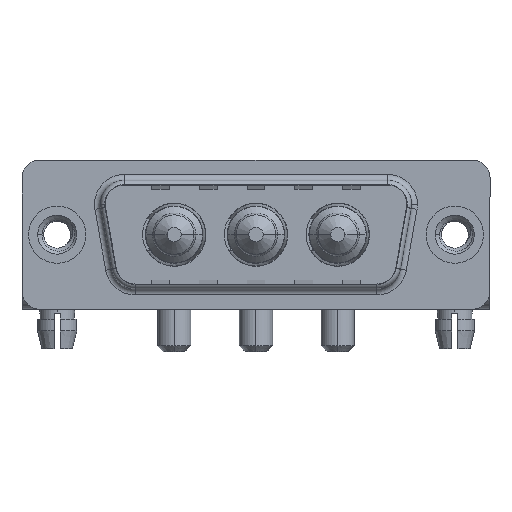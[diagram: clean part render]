
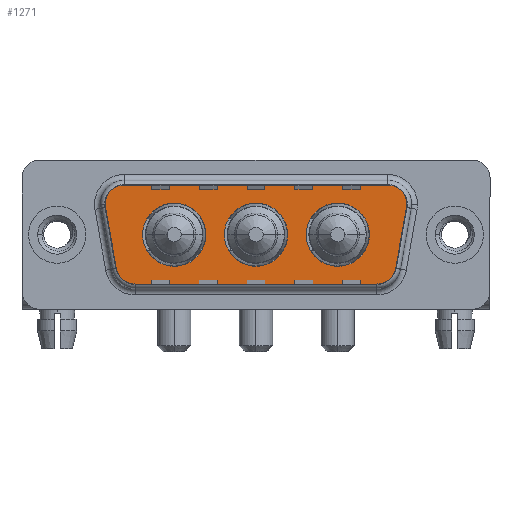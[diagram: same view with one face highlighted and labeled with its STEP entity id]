
A CAD part, top view. The second image highlights one B-rep face of the part: STEP entity #1271.
In plain terms, the highlighted planar face has unit normal (0, 0, 1).
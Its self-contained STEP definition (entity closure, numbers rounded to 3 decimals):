
#171 = VERTEX_POINT ( 'NONE', #11908 ) ;
#190 = CIRCLE ( 'NONE', #13988, 2.65 ) ;
#229 = DIRECTION ( 'NONE',  ( 0., 0., 1. ) ) ;
#417 = DIRECTION ( 'NONE',  ( 0.174, 0.985, 0. ) ) ;
#504 = CARTESIAN_POINT ( 'NONE',  ( 26.866, -2.9, 0. ) ) ;
#672 = CARTESIAN_POINT ( 'NONE',  ( 14., 0., 0. ) ) ;
#733 = CARTESIAN_POINT ( 'NONE',  ( 6.434, -4.9, 0. ) ) ;
#956 = ORIENTED_EDGE ( 'NONE', *, *, #7498, .F. ) ;
#975 = CARTESIAN_POINT ( 'NONE',  ( 5.411, 4.9, 0. ) ) ;
#1110 = EDGE_CURVE ( 'NONE', #8592, #13271, #4122, .T. ) ;
#1236 = LINE ( 'NONE', #11989, #11719 ) ;
#1271 = ADVANCED_FACE ( 'NONE', ( #8222, #8380, #13931, #12804 ), #3369, .T. ) ;
#1402 = VERTEX_POINT ( 'NONE', #4057 ) ;
#1997 = EDGE_LOOP ( 'NONE', ( #13132, #956 ) ) ;
#2053 = CIRCLE ( 'NONE', #6487, 2.65 ) ;
#2118 = VERTEX_POINT ( 'NONE', #13344 ) ;
#2180 = EDGE_CURVE ( 'NONE', #5391, #5598, #190, .T. ) ;
#2193 = ORIENTED_EDGE ( 'NONE', *, *, #7189, .F. ) ;
#2213 = DIRECTION ( 'NONE',  ( 1., 0., 0. ) ) ;
#2269 = CIRCLE ( 'NONE', #9163, 2. ) ;
#2426 = EDGE_CURVE ( 'NONE', #1402, #171, #12169, .T. ) ;
#2434 = CARTESIAN_POINT ( 'NONE',  ( 29.889, 2.9, 0. ) ) ;
#2473 = LINE ( 'NONE', #10884, #14920 ) ;
#2818 = AXIS2_PLACEMENT_3D ( 'NONE', #11722, #11875, #3447 ) ;
#2893 = ORIENTED_EDGE ( 'NONE', *, *, #14145, .T. ) ;
#3054 = CIRCLE ( 'NONE', #2818, 2.65 ) ;
#3228 = CARTESIAN_POINT ( 'NONE',  ( 20.85, 0., 0. ) ) ;
#3335 = DIRECTION ( 'NONE',  ( 0., 0., 1. ) ) ;
#3369 = PLANE ( 'NONE',  #13963 ) ;
#3447 = DIRECTION ( 'NONE',  ( 1., 0., 0. ) ) ;
#3895 = DIRECTION ( 'NONE',  ( 0., 0., 1. ) ) ;
#3896 = DIRECTION ( 'NONE',  ( 0., 0., 1. ) ) ;
#3942 = ORIENTED_EDGE ( 'NONE', *, *, #14695, .T. ) ;
#4038 = DIRECTION ( 'NONE',  ( 1., 0., 0. ) ) ;
#4057 = CARTESIAN_POINT ( 'NONE',  ( 28.836, -3.247, 0. ) ) ;
#4072 = DIRECTION ( 'NONE',  ( 0., 0., 1. ) ) ;
#4122 = CIRCLE ( 'NONE', #11779, 2. ) ;
#4148 = LINE ( 'NONE', #8859, #6401 ) ;
#4158 = VERTEX_POINT ( 'NONE', #733 ) ;
#4188 = EDGE_CURVE ( 'NONE', #4158, #2118, #4148, .T. ) ;
#4205 = CARTESIAN_POINT ( 'NONE',  ( 29.859, 2.553, 0. ) ) ;
#4219 = EDGE_CURVE ( 'NONE', #2118, #1402, #6156, .T. ) ;
#4650 = ORIENTED_EDGE ( 'NONE', *, *, #1110, .T. ) ;
#4975 = DIRECTION ( 'NONE',  ( 1., 0., 0. ) ) ;
#5220 = ORIENTED_EDGE ( 'NONE', *, *, #10240, .T. ) ;
#5391 = VERTEX_POINT ( 'NONE', #13229 ) ;
#5438 = VERTEX_POINT ( 'NONE', #10531 ) ;
#5490 = DIRECTION ( 'NONE',  ( 0., 0., 1. ) ) ;
#5598 = VERTEX_POINT ( 'NONE', #8586 ) ;
#5659 = DIRECTION ( 'NONE',  ( -1., 0., 0. ) ) ;
#5810 = DIRECTION ( 'NONE',  ( 1., 0., 0. ) ) ;
#5911 = VERTEX_POINT ( 'NONE', #7251 ) ;
#5928 = EDGE_LOOP ( 'NONE', ( #13941, #7519, #6451, #2893, #3942, #4650, #14948, #5220, #11555 ) ) ;
#5951 = DIRECTION ( 'NONE',  ( 0.174, -0.985, 0. ) ) ;
#6156 = CIRCLE ( 'NONE', #12092, 2. ) ;
#6262 = AXIS2_PLACEMENT_3D ( 'NONE', #8022, #5490, #9117 ) ;
#6385 = CARTESIAN_POINT ( 'NONE',  ( 9.8, 0., 0. ) ) ;
#6401 = VECTOR ( 'NONE', #9788, 1000. ) ;
#6451 = ORIENTED_EDGE ( 'NONE', *, *, #11445, .T. ) ;
#6487 = AXIS2_PLACEMENT_3D ( 'NONE', #9053, #10300, #5810 ) ;
#6746 = DIRECTION ( 'NONE',  ( 1., 0., 0. ) ) ;
#6749 = AXIS2_PLACEMENT_3D ( 'NONE', #15021, #12638, #6746 ) ;
#7189 = EDGE_CURVE ( 'NONE', #15166, #12418, #12930, .T. ) ;
#7204 = CIRCLE ( 'NONE', #9674, 2. ) ;
#7251 = CARTESIAN_POINT ( 'NONE',  ( 19.3, 0., 0. ) ) ;
#7318 = DIRECTION ( 'NONE',  ( 1., 0., 0. ) ) ;
#7381 = VERTEX_POINT ( 'NONE', #672 ) ;
#7498 = EDGE_CURVE ( 'NONE', #5598, #5391, #3054, .T. ) ;
#7519 = ORIENTED_EDGE ( 'NONE', *, *, #2426, .T. ) ;
#7532 = VERTEX_POINT ( 'NONE', #8072 ) ;
#7845 = ORIENTED_EDGE ( 'NONE', *, *, #9099, .F. ) ;
#8022 = CARTESIAN_POINT ( 'NONE',  ( 27.889, 2.9, 0. ) ) ;
#8066 = CARTESIAN_POINT ( 'NONE',  ( 26.866, -2.9, 0. ) ) ;
#8072 = CARTESIAN_POINT ( 'NONE',  ( 27.889, 4.9, 0. ) ) ;
#8177 = EDGE_LOOP ( 'NONE', ( #7845, #2193 ) ) ;
#8222 = FACE_BOUND ( 'NONE', #12948, .T. ) ;
#8380 = FACE_BOUND ( 'NONE', #8177, .T. ) ;
#8495 = CIRCLE ( 'NONE', #6262, 2. ) ;
#8586 = CARTESIAN_POINT ( 'NONE',  ( 7.15, 0., 0. ) ) ;
#8592 = VERTEX_POINT ( 'NONE', #975 ) ;
#8859 = CARTESIAN_POINT ( 'NONE',  ( 6.434, -4.9, 0. ) ) ;
#9053 = CARTESIAN_POINT ( 'NONE',  ( 16.65, 0., 0. ) ) ;
#9099 = EDGE_CURVE ( 'NONE', #12418, #15166, #14637, .T. ) ;
#9117 = DIRECTION ( 'NONE',  ( -1., 0., 0. ) ) ;
#9163 = AXIS2_PLACEMENT_3D ( 'NONE', #9759, #3896, #10918 ) ;
#9596 = EDGE_CURVE ( 'NONE', #13271, #5438, #1236, .T. ) ;
#9674 = AXIS2_PLACEMENT_3D ( 'NONE', #12546, #3335, #5659 ) ;
#9726 = DIRECTION ( 'NONE',  ( -1., 0., 0. ) ) ;
#9759 = CARTESIAN_POINT ( 'NONE',  ( 27.889, 2.9, 0. ) ) ;
#9788 = DIRECTION ( 'NONE',  ( 1., 0., 0. ) ) ;
#10240 = EDGE_CURVE ( 'NONE', #5438, #4158, #7204, .T. ) ;
#10300 = DIRECTION ( 'NONE',  ( 0., 0., 1. ) ) ;
#10531 = CARTESIAN_POINT ( 'NONE',  ( 4.464, -3.247, 0. ) ) ;
#10884 = CARTESIAN_POINT ( 'NONE',  ( 5.411, 4.9, 0. ) ) ;
#10918 = DIRECTION ( 'NONE',  ( -1., 0., 0. ) ) ;
#11262 = DIRECTION ( 'NONE',  ( 1., 0., 0. ) ) ;
#11284 = VERTEX_POINT ( 'NONE', #2434 ) ;
#11445 = EDGE_CURVE ( 'NONE', #171, #11284, #2269, .T. ) ;
#11555 = ORIENTED_EDGE ( 'NONE', *, *, #4188, .T. ) ;
#11571 = VECTOR ( 'NONE', #417, 1000. ) ;
#11675 = ORIENTED_EDGE ( 'NONE', *, *, #13079, .F. ) ;
#11700 = AXIS2_PLACEMENT_3D ( 'NONE', #12384, #3895, #4038 ) ;
#11719 = VECTOR ( 'NONE', #5951, 1000. ) ;
#11722 = CARTESIAN_POINT ( 'NONE',  ( 9.8, 0., 0. ) ) ;
#11779 = AXIS2_PLACEMENT_3D ( 'NONE', #14796, #13640, #2213 ) ;
#11812 = EDGE_CURVE ( 'NONE', #7381, #5911, #14254, .T. ) ;
#11875 = DIRECTION ( 'NONE',  ( 0., 0., 1. ) ) ;
#11908 = CARTESIAN_POINT ( 'NONE',  ( 29.859, 2.553, 0. ) ) ;
#11989 = CARTESIAN_POINT ( 'NONE',  ( 3.441, 2.553, 0. ) ) ;
#12076 = CARTESIAN_POINT ( 'NONE',  ( 3.441, 2.553, 0. ) ) ;
#12092 = AXIS2_PLACEMENT_3D ( 'NONE', #504, #4072, #11262 ) ;
#12169 = LINE ( 'NONE', #4205, #11571 ) ;
#12384 = CARTESIAN_POINT ( 'NONE',  ( 23.5, 0., 0. ) ) ;
#12418 = VERTEX_POINT ( 'NONE', #15203 ) ;
#12546 = CARTESIAN_POINT ( 'NONE',  ( 6.434, -2.9, 0. ) ) ;
#12638 = DIRECTION ( 'NONE',  ( 0., 0., 1. ) ) ;
#12804 = FACE_OUTER_BOUND ( 'NONE', #5928, .T. ) ;
#12930 = CIRCLE ( 'NONE', #11700, 2.65 ) ;
#12948 = EDGE_LOOP ( 'NONE', ( #11675, #14486 ) ) ;
#13079 = EDGE_CURVE ( 'NONE', #5911, #7381, #2053, .T. ) ;
#13132 = ORIENTED_EDGE ( 'NONE', *, *, #2180, .F. ) ;
#13139 = DIRECTION ( 'NONE',  ( 1., 0., 0. ) ) ;
#13171 = DIRECTION ( 'NONE',  ( 0., 0., 1. ) ) ;
#13229 = CARTESIAN_POINT ( 'NONE',  ( 12.45, 0., 0. ) ) ;
#13271 = VERTEX_POINT ( 'NONE', #12076 ) ;
#13344 = CARTESIAN_POINT ( 'NONE',  ( 26.866, -4.9, 0. ) ) ;
#13568 = DIRECTION ( 'NONE',  ( 0., 0., 1. ) ) ;
#13640 = DIRECTION ( 'NONE',  ( 0., 0., 1. ) ) ;
#13931 = FACE_BOUND ( 'NONE', #1997, .T. ) ;
#13941 = ORIENTED_EDGE ( 'NONE', *, *, #4219, .T. ) ;
#13963 = AXIS2_PLACEMENT_3D ( 'NONE', #8066, #13171, #4975 ) ;
#13988 = AXIS2_PLACEMENT_3D ( 'NONE', #6385, #13568, #7318 ) ;
#14122 = CARTESIAN_POINT ( 'NONE',  ( 16.65, 0., 0. ) ) ;
#14145 = EDGE_CURVE ( 'NONE', #11284, #7532, #8495, .T. ) ;
#14254 = CIRCLE ( 'NONE', #14510, 2.65 ) ;
#14486 = ORIENTED_EDGE ( 'NONE', *, *, #11812, .F. ) ;
#14510 = AXIS2_PLACEMENT_3D ( 'NONE', #14122, #229, #13139 ) ;
#14637 = CIRCLE ( 'NONE', #6749, 2.65 ) ;
#14695 = EDGE_CURVE ( 'NONE', #7532, #8592, #2473, .T. ) ;
#14796 = CARTESIAN_POINT ( 'NONE',  ( 5.411, 2.9, 0. ) ) ;
#14920 = VECTOR ( 'NONE', #9726, 1000. ) ;
#14948 = ORIENTED_EDGE ( 'NONE', *, *, #9596, .T. ) ;
#15021 = CARTESIAN_POINT ( 'NONE',  ( 23.5, 0., 0. ) ) ;
#15166 = VERTEX_POINT ( 'NONE', #3228 ) ;
#15203 = CARTESIAN_POINT ( 'NONE',  ( 26.15, 0., 0. ) ) ;
